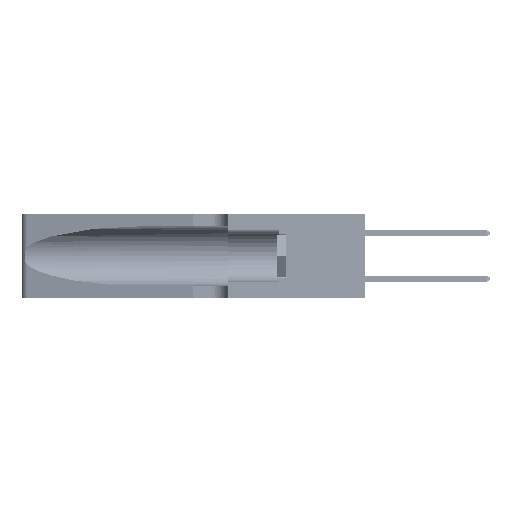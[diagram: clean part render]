
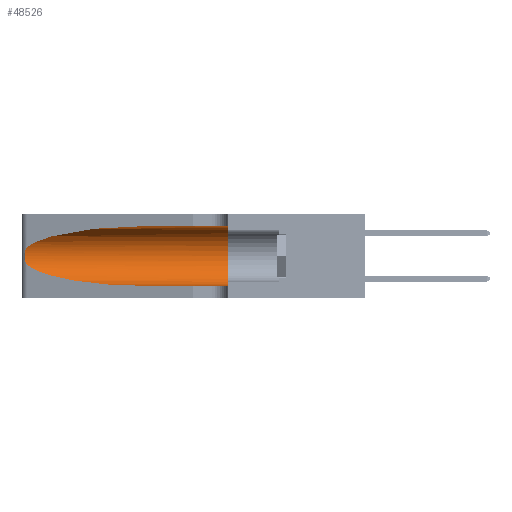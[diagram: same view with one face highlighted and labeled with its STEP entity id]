
A CAD part, left-side view. The second image highlights one B-rep face of the part: STEP entity #48526.
In plain terms, the highlighted cylindrical face has radius 3.308 mm (diameter 6.617 mm), a partial arc.
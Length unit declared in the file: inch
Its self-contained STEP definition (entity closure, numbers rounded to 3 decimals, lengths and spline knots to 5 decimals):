
#466 = VERTEX_POINT ( 'NONE', #29931 ) ;
#684 = CARTESIAN_POINT ( 'NONE',  ( 0.25639, 1.23184, 0.21858 ) ) ;
#781 = DIRECTION ( 'NONE',  ( 0., 0., 1. ) ) ;
#862 = CARTESIAN_POINT ( 'NONE',  ( 0.25789, 1.23486, 0.15765 ) ) ;
#2454 = ORIENTED_EDGE ( 'NONE', *, *, #14927, .T. ) ;
#5001 = CARTESIAN_POINT ( 'NONE',  ( 0.25555, 1.22993, 0.14849 ) ) ;
#5375 = CARTESIAN_POINT ( 'NONE',  ( 0.1305, 0.35, 0.31525 ) ) ;
#5523 = ORIENTED_EDGE ( 'NONE', *, *, #46610, .F. ) ;
#6429 = VECTOR ( 'NONE', #48382, 39.37008 ) ;
#7699 = LINE ( 'NONE', #11295, #6429 ) ;
#9672 = CARTESIAN_POINT ( 'NONE',  ( 0.18966, 0.96281, 0.31525 ) ) ;
#10285 = ORIENTED_EDGE ( 'NONE', *, *, #47540, .T. ) ;
#10952 = VERTEX_POINT ( 'NONE', #53221 ) ;
#11295 = CARTESIAN_POINT ( 'NONE',  ( 0.1305, 1.61858, 0.31525 ) ) ;
#12888 = ORIENTED_EDGE ( 'NONE', *, *, #38621, .T. ) ;
#12957 = DIRECTION ( 'NONE',  ( 0., 0., -1. ) ) ;
#13111 = CARTESIAN_POINT ( 'NONE',  ( 0.25787, 1.23484, 0.2124 ) ) ;
#13965 = CARTESIAN_POINT ( 'NONE',  ( 0.25487, 1.22718, 0.22369 ) ) ;
#14927 = EDGE_CURVE ( 'NONE', #29172, #28551, #21047, .T. ) ;
#17242 = CARTESIAN_POINT ( 'NONE',  ( 0.26018, 1.23835, 0.19895 ) ) ;
#18096 = CARTESIAN_POINT ( 'NONE',  ( 0.25487, 1.22718, 0.22369 ) ) ;
#18472 = VECTOR ( 'NONE', #22651, 39.37008 ) ;
#21047 = B_SPLINE_CURVE_WITH_KNOTS ( 'NONE', 3,
 ( #37751, #45877, #684, #13111, #41901, #17242, #46052, #21383, #50183, #25509, #862, #29674, #5001, #33783 ),
 .UNSPECIFIED., .F., .F.,
 ( 4, 2, 2, 2, 2, 2, 4 ),
 ( 0., 0.00027, 0.00053, 0.00107, 0.0016, 0.00187, 0.00214 ),
 .UNSPECIFIED. ) ;
#21162 = CIRCLE ( 'NONE', #26530, 0.13025 ) ;
#21383 = CARTESIAN_POINT ( 'NONE',  ( 0.26075, 1.23896, 0.178 ) ) ;
#22101 = EDGE_LOOP ( 'NONE', ( #12888, #2454, #25289, #10285, #5523, #23175 ) ) ;
#22639 = CARTESIAN_POINT ( 'NONE',  ( 0.25487, 1.22718, 0.14631 ) ) ;
#22651 = DIRECTION ( 'NONE',  ( 0., -1., 0. ) ) ;
#23175 = ORIENTED_EDGE ( 'NONE', *, *, #24249, .F. ) ;
#23915 = EDGE_CURVE ( 'NONE', #28551, #50337, #47890, .T. ) ;
#24134 = CYLINDRICAL_SURFACE ( 'NONE', #27669, 0.13025 ) ;
#24249 = EDGE_CURVE ( 'NONE', #466, #52684, #7699, .T. ) ;
#25191 = DIRECTION ( 'NONE',  ( 0., -1., 0. ) ) ;
#25289 = ORIENTED_EDGE ( 'NONE', *, *, #23915, .T. ) ;
#25422 = DIRECTION ( 'NONE',  ( 0., 1., 0. ) ) ;
#25509 = CARTESIAN_POINT ( 'NONE',  ( 0.25856, 1.23593, 0.16098 ) ) ;
#26336 = CARTESIAN_POINT ( 'NONE',  ( 0.1305, 0.72297, 0.05475 ) ) ;
#26530 = AXIS2_PLACEMENT_3D ( 'NONE', #50103, #25422, #781 ) ;
#27669 = AXIS2_PLACEMENT_3D ( 'NONE', #37612, #25191, #12957 ) ;
#28551 = VERTEX_POINT ( 'NONE', #22639 ) ;
#29172 = VERTEX_POINT ( 'NONE', #18096 ) ;
#29189 = CARTESIAN_POINT ( 'NONE',  ( 0.1305, 0.72297, 0.05475 ) ) ;
#29674 = CARTESIAN_POINT ( 'NONE',  ( 0.25639, 1.23186, 0.15144 ) ) ;
#29931 = CARTESIAN_POINT ( 'NONE',  ( 0.1305, 0.72297, 0.31525 ) ) ;
#33783 = CARTESIAN_POINT ( 'NONE',  ( 0.25487, 1.22718, 0.14631 ) ) ;
#34433 = CARTESIAN_POINT ( 'NONE',  ( 0.2373, 1.15595, 0.08982 ) ) ;
#37612 = CARTESIAN_POINT ( 'NONE',  ( 0.1305, 1.61858, 0.185 ) ) ;
#37751 = CARTESIAN_POINT ( 'NONE',  ( 0.25487, 1.22718, 0.22369 ) ) ;
#38619 = CARTESIAN_POINT ( 'NONE',  ( 0.2373, 1.15595, 0.28018 ) ) ;
#38621 = EDGE_CURVE ( 'NONE', #466, #29172, #50863, .T. ) ;
#41901 = CARTESIAN_POINT ( 'NONE',  ( 0.25854, 1.2359, 0.20912 ) ) ;
#45877 = CARTESIAN_POINT ( 'NONE',  ( 0.25555, 1.22994, 0.2215 ) ) ;
#46052 = CARTESIAN_POINT ( 'NONE',  ( 0.26075, 1.23896, 0.19203 ) ) ;
#46068 = FACE_OUTER_BOUND ( 'NONE', #22101, .T. ) ;
#46610 = EDGE_CURVE ( 'NONE', #52684, #10952, #21162, .T. ) ;
#46866 = CARTESIAN_POINT ( 'NONE',  ( 0.25487, 1.22718, 0.14631 ) ) ;
#47540 = EDGE_CURVE ( 'NONE', #50337, #10952, #51332, .T. ) ;
#47890 =( BOUNDED_CURVE ( )  B_SPLINE_CURVE ( 3, ( #46866, #34433, #51016, #26336 ),
 .UNSPECIFIED., .F., .F. ) 
 B_SPLINE_CURVE_WITH_KNOTS ( ( 4, 4 ),
 ( 3.44316, 4.71239 ),
 .UNSPECIFIED. ) 
 CURVE ( )  GEOMETRIC_REPRESENTATION_ITEM ( )  RATIONAL_B_SPLINE_CURVE ( ( 1., 0.87, 0.87, 1. ) ) 
 REPRESENTATION_ITEM ( '' )  );
#48382 = DIRECTION ( 'NONE',  ( 0., -1., 0. ) ) ;
#48526 = ADVANCED_FACE ( 'NONE', ( #46068 ), #24134, .F. ) ;
#50103 = CARTESIAN_POINT ( 'NONE',  ( 0.1305, 0.35, 0.185 ) ) ;
#50183 = CARTESIAN_POINT ( 'NONE',  ( 0.26017, 1.23833, 0.17102 ) ) ;
#50337 = VERTEX_POINT ( 'NONE', #29189 ) ;
#50863 =( BOUNDED_CURVE ( )  B_SPLINE_CURVE ( 3, ( #50892, #9672, #38619, #13965 ),
 .UNSPECIFIED., .F., .T. ) 
 B_SPLINE_CURVE_WITH_KNOTS ( ( 4, 4 ),
 ( 1.5708, 2.84003 ),
 .UNSPECIFIED. ) 
 CURVE ( )  GEOMETRIC_REPRESENTATION_ITEM ( )  RATIONAL_B_SPLINE_CURVE ( ( 1., 0.87, 0.87, 1. ) ) 
 REPRESENTATION_ITEM ( '' )  );
#50892 = CARTESIAN_POINT ( 'NONE',  ( 0.1305, 0.72297, 0.31525 ) ) ;
#51016 = CARTESIAN_POINT ( 'NONE',  ( 0.18966, 0.96281, 0.05475 ) ) ;
#51332 = LINE ( 'NONE', #51460, #18472 ) ;
#51460 = CARTESIAN_POINT ( 'NONE',  ( 0.1305, 1.61858, 0.05475 ) ) ;
#52684 = VERTEX_POINT ( 'NONE', #5375 ) ;
#53221 = CARTESIAN_POINT ( 'NONE',  ( 0.1305, 0.35, 0.05475 ) ) ;
